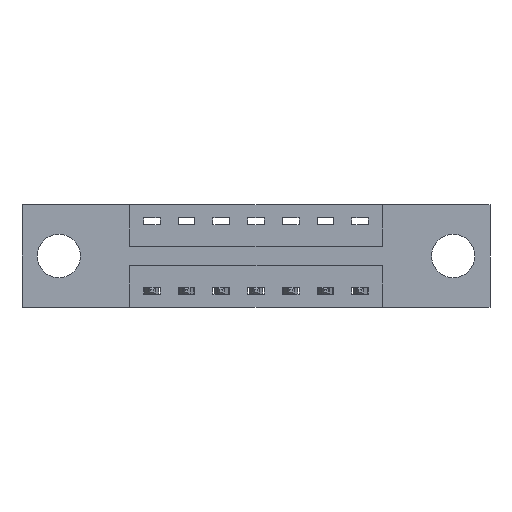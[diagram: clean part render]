
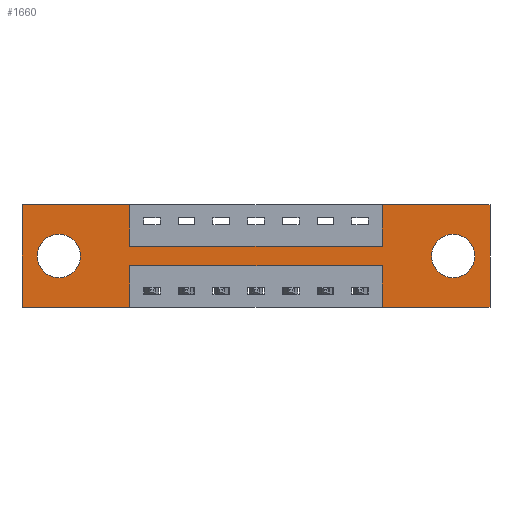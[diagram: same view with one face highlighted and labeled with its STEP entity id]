
A CAD part, front view. The second image highlights one B-rep face of the part: STEP entity #1660.
In plain terms, the highlighted planar face has unit normal (0, -1, 0).
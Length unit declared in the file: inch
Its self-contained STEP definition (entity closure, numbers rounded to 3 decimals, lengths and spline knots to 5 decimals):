
#28 = VECTOR ( 'NONE', #137, 39.37008 ) ;
#74 = CARTESIAN_POINT ( 'NONE',  ( 0., 0., 0. ) ) ;
#137 = DIRECTION ( 'NONE',  ( 0., 0., -1. ) ) ;
#229 = CARTESIAN_POINT ( 'NONE',  ( 0., 0., 0. ) ) ;
#240 = DIRECTION ( 'NONE',  ( 0., 0., -1. ) ) ;
#564 = ORIENTED_EDGE ( 'NONE', *, *, #2200, .T. ) ;
#616 = CARTESIAN_POINT ( 'NONE',  ( 1.5525, 0., -0.107 ) ) ;
#665 = ORIENTED_EDGE ( 'NONE', *, *, #1123, .T. ) ;
#705 = DIRECTION ( 'NONE',  ( -1., 0., 0. ) ) ;
#720 = DIRECTION ( 'NONE',  ( 0., 1., 0. ) ) ;
#771 = CARTESIAN_POINT ( 'NONE',  ( 0., 0., -0.37 ) ) ;
#780 = DIRECTION ( 'NONE',  ( 1., 0., 0. ) ) ;
#785 = VERTEX_POINT ( 'NONE', #8897 ) ;
#899 = CARTESIAN_POINT ( 'NONE',  ( 0.3875, 0., -0.15 ) ) ;
#1101 = CARTESIAN_POINT ( 'NONE',  ( 0.3875, 0., -0.37 ) ) ;
#1123 = EDGE_CURVE ( 'NONE', #8679, #5677, #7824, .T. ) ;
#1127 = DIRECTION ( 'NONE',  ( -1., 0., 0. ) ) ;
#1185 = EDGE_LOOP ( 'NONE', ( #665, #2614 ) ) ;
#1246 = ORIENTED_EDGE ( 'NONE', *, *, #6715, .F. ) ;
#1374 = ORIENTED_EDGE ( 'NONE', *, *, #8600, .F. ) ;
#1410 = DIRECTION ( 'NONE',  ( 0., 0., -1. ) ) ;
#1441 = VERTEX_POINT ( 'NONE', #5892 ) ;
#1477 = DIRECTION ( 'NONE',  ( 0., -1., 0. ) ) ;
#1527 = AXIS2_PLACEMENT_3D ( 'NONE', #5758, #1477, #6447 ) ;
#1590 = CARTESIAN_POINT ( 'NONE',  ( 1.5525, 0., -0.263 ) ) ;
#1660 = ADVANCED_FACE ( 'NONE', ( #9074, #1759, #5325 ), #5725, .T. ) ;
#1759 = FACE_BOUND ( 'NONE', #6117, .T. ) ;
#1770 = DIRECTION ( 'NONE',  ( 0., 0., 1. ) ) ;
#1787 = CARTESIAN_POINT ( 'NONE',  ( 1.2975, 0., -0.37 ) ) ;
#1800 = CARTESIAN_POINT ( 'NONE',  ( 1.685, 0., -0.37 ) ) ;
#1954 = AXIS2_PLACEMENT_3D ( 'NONE', #3536, #8265, #4233 ) ;
#1977 = CARTESIAN_POINT ( 'NONE',  ( 1.2975, 0., -0.15 ) ) ;
#2031 = ORIENTED_EDGE ( 'NONE', *, *, #5684, .F. ) ;
#2044 = ORIENTED_EDGE ( 'NONE', *, *, #2334, .F. ) ;
#2113 = ORIENTED_EDGE ( 'NONE', *, *, #5487, .F. ) ;
#2200 = EDGE_CURVE ( 'NONE', #2636, #785, #5722, .T. ) ;
#2305 = VECTOR ( 'NONE', #240, 39.37008 ) ;
#2329 = VECTOR ( 'NONE', #6421, 39.37008 ) ;
#2334 = EDGE_CURVE ( 'NONE', #7948, #6968, #7602, .T. ) ;
#2341 = CARTESIAN_POINT ( 'NONE',  ( 1.2975, 0., 0. ) ) ;
#2354 = CARTESIAN_POINT ( 'NONE',  ( 1.2975, 0., -0.22 ) ) ;
#2391 = EDGE_CURVE ( 'NONE', #785, #2636, #4970, .T. ) ;
#2500 = EDGE_CURVE ( 'NONE', #7078, #6981, #5514, .T. ) ;
#2614 = ORIENTED_EDGE ( 'NONE', *, *, #7898, .T. ) ;
#2636 = VERTEX_POINT ( 'NONE', #2866 ) ;
#2866 = CARTESIAN_POINT ( 'NONE',  ( 0.1325, 0., -0.263 ) ) ;
#2934 = ORIENTED_EDGE ( 'NONE', *, *, #8964, .F. ) ;
#3037 = VERTEX_POINT ( 'NONE', #4037 ) ;
#3162 = DIRECTION ( 'NONE',  ( 1., 0., 0. ) ) ;
#3247 = CARTESIAN_POINT ( 'NONE',  ( 0., 0., 0. ) ) ;
#3402 = EDGE_CURVE ( 'NONE', #8137, #7569, #3642, .T. ) ;
#3536 = CARTESIAN_POINT ( 'NONE',  ( 0.1325, 0., -0.185 ) ) ;
#3566 = CARTESIAN_POINT ( 'NONE',  ( 0., 0., 0. ) ) ;
#3642 = LINE ( 'NONE', #8590, #5279 ) ;
#3660 = VECTOR ( 'NONE', #1127, 39.37008 ) ;
#3917 = CARTESIAN_POINT ( 'NONE',  ( 0.1325, 0., -0.185 ) ) ;
#3976 = ORIENTED_EDGE ( 'NONE', *, *, #2500, .F. ) ;
#4037 = CARTESIAN_POINT ( 'NONE',  ( 0., 0., -0.37 ) ) ;
#4096 = ORIENTED_EDGE ( 'NONE', *, *, #7874, .F. ) ;
#4128 = LINE ( 'NONE', #5017, #7724 ) ;
#4137 = EDGE_CURVE ( 'NONE', #6968, #4142, #7767, .T. ) ;
#4142 = VERTEX_POINT ( 'NONE', #1800 ) ;
#4204 = LINE ( 'NONE', #4388, #2329 ) ;
#4233 = DIRECTION ( 'NONE',  ( 0., 0., 1. ) ) ;
#4277 = CARTESIAN_POINT ( 'NONE',  ( 1.2975, 0., 0. ) ) ;
#4335 = VECTOR ( 'NONE', #4989, 39.37008 ) ;
#4388 = CARTESIAN_POINT ( 'NONE',  ( 0., 0., -0.37 ) ) ;
#4562 = EDGE_LOOP ( 'NONE', ( #2934, #3976, #5947, #4096, #7314, #2044, #8711, #4865, #2113, #1246, #1374, #2031 ) ) ;
#4606 = AXIS2_PLACEMENT_3D ( 'NONE', #5115, #720, #5815 ) ;
#4624 = CARTESIAN_POINT ( 'NONE',  ( 1.2975, 0., -0.37 ) ) ;
#4633 = DIRECTION ( 'NONE',  ( 0., 0., 1. ) ) ;
#4865 = ORIENTED_EDGE ( 'NONE', *, *, #3402, .F. ) ;
#4871 = DIRECTION ( 'NONE',  ( 0., 0., -1. ) ) ;
#4929 = AXIS2_PLACEMENT_3D ( 'NONE', #3917, #8652, #4633 ) ;
#4970 = CIRCLE ( 'NONE', #4929, 0.078 ) ;
#4989 = DIRECTION ( 'NONE',  ( 0., 0., 1. ) ) ;
#5017 = CARTESIAN_POINT ( 'NONE',  ( 0.3875, 0., 0. ) ) ;
#5027 = VERTEX_POINT ( 'NONE', #229 ) ;
#5035 = VERTEX_POINT ( 'NONE', #1787 ) ;
#5084 = VECTOR ( 'NONE', #8666, 39.37008 ) ;
#5115 = CARTESIAN_POINT ( 'NONE',  ( 1.5525, 0., -0.185 ) ) ;
#5279 = VECTOR ( 'NONE', #3162, 39.37008 ) ;
#5325 = FACE_OUTER_BOUND ( 'NONE', #4562, .T. ) ;
#5439 = EDGE_CURVE ( 'NONE', #7569, #7948, #7930, .T. ) ;
#5446 = DIRECTION ( 'NONE',  ( 0., 1., 0. ) ) ;
#5456 = CARTESIAN_POINT ( 'NONE',  ( 1.5525, 0., -0.185 ) ) ;
#5487 = EDGE_CURVE ( 'NONE', #1441, #8137, #4128, .T. ) ;
#5514 = LINE ( 'NONE', #6832, #3660 ) ;
#5677 = VERTEX_POINT ( 'NONE', #1590 ) ;
#5684 = EDGE_CURVE ( 'NONE', #8328, #3037, #8236, .T. ) ;
#5722 = CIRCLE ( 'NONE', #1954, 0.078 ) ;
#5725 = PLANE ( 'NONE',  #1527 ) ;
#5729 = CARTESIAN_POINT ( 'NONE',  ( 1.685, 0., 0. ) ) ;
#5758 = CARTESIAN_POINT ( 'NONE',  ( 0., 0., -0.37 ) ) ;
#5797 = LINE ( 'NONE', #7229, #28 ) ;
#5815 = DIRECTION ( 'NONE',  ( 0., 0., -1. ) ) ;
#5820 = CIRCLE ( 'NONE', #4606, 0.078 ) ;
#5829 = VECTOR ( 'NONE', #780, 39.37008 ) ;
#5892 = CARTESIAN_POINT ( 'NONE',  ( 0.3875, 0., 0. ) ) ;
#5947 = ORIENTED_EDGE ( 'NONE', *, *, #7289, .F. ) ;
#6025 = AXIS2_PLACEMENT_3D ( 'NONE', #5456, #5446, #4871 ) ;
#6117 = EDGE_LOOP ( 'NONE', ( #8014, #564 ) ) ;
#6292 = VECTOR ( 'NONE', #705, 39.37008 ) ;
#6421 = DIRECTION ( 'NONE',  ( -1., 0., 0. ) ) ;
#6447 = DIRECTION ( 'NONE',  ( 0., 0., -1. ) ) ;
#6467 = LINE ( 'NONE', #4624, #8010 ) ;
#6548 = LINE ( 'NONE', #3566, #8099 ) ;
#6715 = EDGE_CURVE ( 'NONE', #5027, #1441, #8651, .T. ) ;
#6832 = CARTESIAN_POINT ( 'NONE',  ( 0.3875, 0., -0.22 ) ) ;
#6968 = VERTEX_POINT ( 'NONE', #5729 ) ;
#6981 = VERTEX_POINT ( 'NONE', #7741 ) ;
#7078 = VERTEX_POINT ( 'NONE', #2354 ) ;
#7229 = CARTESIAN_POINT ( 'NONE',  ( 0.3875, 0., -0.37 ) ) ;
#7289 = EDGE_CURVE ( 'NONE', #5035, #7078, #6467, .T. ) ;
#7314 = ORIENTED_EDGE ( 'NONE', *, *, #4137, .F. ) ;
#7569 = VERTEX_POINT ( 'NONE', #1977 ) ;
#7602 = LINE ( 'NONE', #74, #5829 ) ;
#7636 = DIRECTION ( 'NONE',  ( 0., 0., 1. ) ) ;
#7724 = VECTOR ( 'NONE', #1410, 39.37008 ) ;
#7741 = CARTESIAN_POINT ( 'NONE',  ( 0.3875, 0., -0.22 ) ) ;
#7767 = LINE ( 'NONE', #7991, #2305 ) ;
#7824 = CIRCLE ( 'NONE', #6025, 0.078 ) ;
#7874 = EDGE_CURVE ( 'NONE', #4142, #5035, #4204, .T. ) ;
#7898 = EDGE_CURVE ( 'NONE', #5677, #8679, #5820, .T. ) ;
#7930 = LINE ( 'NONE', #4277, #4335 ) ;
#7948 = VERTEX_POINT ( 'NONE', #2341 ) ;
#7991 = CARTESIAN_POINT ( 'NONE',  ( 1.685, 0., 0. ) ) ;
#8010 = VECTOR ( 'NONE', #1770, 39.37008 ) ;
#8014 = ORIENTED_EDGE ( 'NONE', *, *, #2391, .T. ) ;
#8099 = VECTOR ( 'NONE', #7636, 39.37008 ) ;
#8137 = VERTEX_POINT ( 'NONE', #899 ) ;
#8236 = LINE ( 'NONE', #771, #6292 ) ;
#8265 = DIRECTION ( 'NONE',  ( 0., 1., 0. ) ) ;
#8328 = VERTEX_POINT ( 'NONE', #1101 ) ;
#8590 = CARTESIAN_POINT ( 'NONE',  ( 0.3875, 0., -0.15 ) ) ;
#8600 = EDGE_CURVE ( 'NONE', #3037, #5027, #6548, .T. ) ;
#8651 = LINE ( 'NONE', #3247, #5084 ) ;
#8652 = DIRECTION ( 'NONE',  ( 0., 1., 0. ) ) ;
#8666 = DIRECTION ( 'NONE',  ( 1., 0., 0. ) ) ;
#8679 = VERTEX_POINT ( 'NONE', #616 ) ;
#8711 = ORIENTED_EDGE ( 'NONE', *, *, #5439, .F. ) ;
#8897 = CARTESIAN_POINT ( 'NONE',  ( 0.1325, 0., -0.107 ) ) ;
#8964 = EDGE_CURVE ( 'NONE', #6981, #8328, #5797, .T. ) ;
#9074 = FACE_BOUND ( 'NONE', #1185, .T. ) ;
